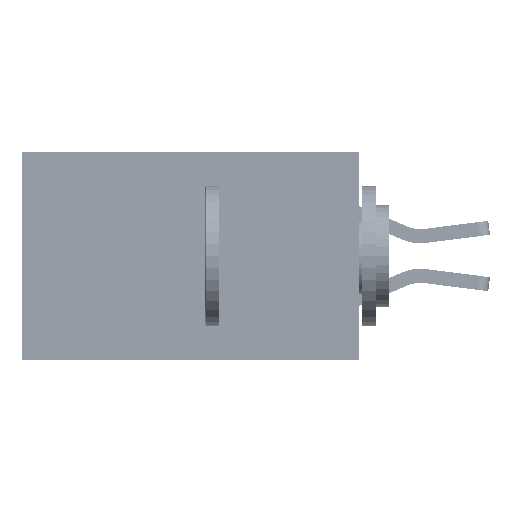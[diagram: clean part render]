
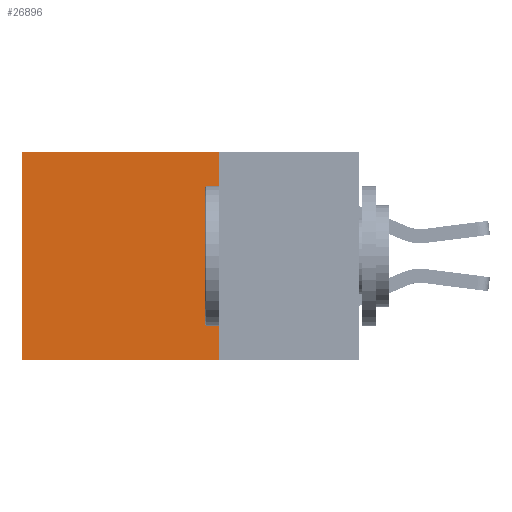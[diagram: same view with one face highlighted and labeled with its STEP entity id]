
A CAD part, left-side view. The second image highlights one B-rep face of the part: STEP entity #26896.
In plain terms, the highlighted planar face has unit normal (-1, 0, 0).
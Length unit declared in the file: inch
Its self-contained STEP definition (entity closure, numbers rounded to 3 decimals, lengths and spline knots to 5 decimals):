
#759 = DIRECTION ( 'NONE',  ( 0., 0., -1. ) ) ;
#2885 = VECTOR ( 'NONE', #10813, 39.37008 ) ;
#4332 = EDGE_LOOP ( 'NONE', ( #38353, #8557, #30146, #28527 ) ) ;
#4521 = FACE_OUTER_BOUND ( 'NONE', #4332, .T. ) ;
#4851 = CARTESIAN_POINT ( 'NONE',  ( 0.2875, 0.25, 0. ) ) ;
#4895 = EDGE_CURVE ( 'NONE', #10603, #37885, #19080, .T. ) ;
#8557 = ORIENTED_EDGE ( 'NONE', *, *, #17747, .F. ) ;
#10603 = VERTEX_POINT ( 'NONE', #36046 ) ;
#10813 = DIRECTION ( 'NONE',  ( 0., 1., 0. ) ) ;
#11600 = PLANE ( 'NONE',  #16435 ) ;
#12083 = CARTESIAN_POINT ( 'NONE',  ( 0.2875, 0.25, -0.37 ) ) ;
#13730 = VECTOR ( 'NONE', #21596, 39.37008 ) ;
#13794 = VERTEX_POINT ( 'NONE', #12083 ) ;
#14624 = LINE ( 'NONE', #23905, #27654 ) ;
#14946 = CARTESIAN_POINT ( 'NONE',  ( 0.2875, 0.6, -0.37 ) ) ;
#15590 = CARTESIAN_POINT ( 'NONE',  ( 0.2875, 0.25, 0. ) ) ;
#16435 = AXIS2_PLACEMENT_3D ( 'NONE', #19536, #24249, #34220 ) ;
#17747 = EDGE_CURVE ( 'NONE', #13794, #37885, #14624, .T. ) ;
#19080 = LINE ( 'NONE', #36193, #23269 ) ;
#19536 = CARTESIAN_POINT ( 'NONE',  ( 0.2875, 0.25, 0. ) ) ;
#20601 = LINE ( 'NONE', #4851, #2885 ) ;
#21596 = DIRECTION ( 'NONE',  ( 0., 0., -1. ) ) ;
#22230 = EDGE_CURVE ( 'NONE', #26126, #13794, #34199, .T. ) ;
#23269 = VECTOR ( 'NONE', #759, 39.37008 ) ;
#23905 = CARTESIAN_POINT ( 'NONE',  ( 0.2875, 0.25, -0.37 ) ) ;
#24249 = DIRECTION ( 'NONE',  ( 1., 0., 0. ) ) ;
#26126 = VERTEX_POINT ( 'NONE', #37090 ) ;
#26896 = ADVANCED_FACE ( 'NONE', ( #4521 ), #11600, .F. ) ;
#26994 = DIRECTION ( 'NONE',  ( 0., 1., 0. ) ) ;
#27654 = VECTOR ( 'NONE', #26994, 39.37008 ) ;
#28527 = ORIENTED_EDGE ( 'NONE', *, *, #33669, .T. ) ;
#30146 = ORIENTED_EDGE ( 'NONE', *, *, #22230, .F. ) ;
#33669 = EDGE_CURVE ( 'NONE', #26126, #10603, #20601, .T. ) ;
#34199 = LINE ( 'NONE', #15590, #13730 ) ;
#34220 = DIRECTION ( 'NONE',  ( 0., 0., -1. ) ) ;
#36046 = CARTESIAN_POINT ( 'NONE',  ( 0.2875, 0.6, 0. ) ) ;
#36193 = CARTESIAN_POINT ( 'NONE',  ( 0.2875, 0.6, 0. ) ) ;
#37090 = CARTESIAN_POINT ( 'NONE',  ( 0.2875, 0.25, 0. ) ) ;
#37885 = VERTEX_POINT ( 'NONE', #14946 ) ;
#38353 = ORIENTED_EDGE ( 'NONE', *, *, #4895, .T. ) ;
